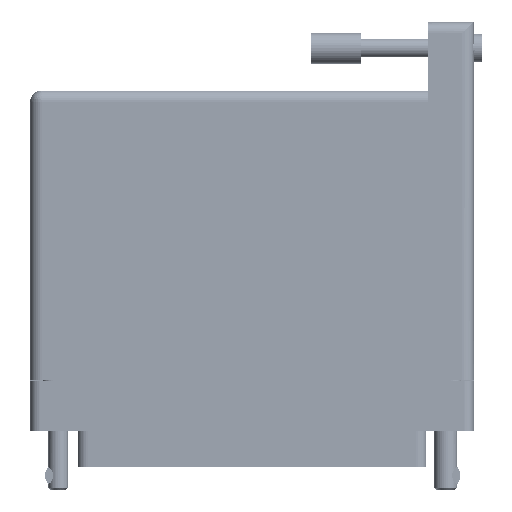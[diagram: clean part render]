
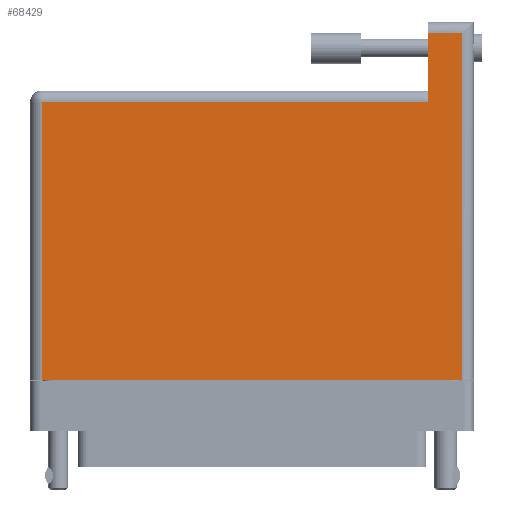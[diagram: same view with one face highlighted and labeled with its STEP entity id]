
A CAD part, front view. The second image highlights one B-rep face of the part: STEP entity #68429.
In plain terms, the highlighted face is planar.
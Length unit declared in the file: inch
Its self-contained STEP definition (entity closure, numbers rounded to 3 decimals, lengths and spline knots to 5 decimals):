
#145 = CARTESIAN_POINT ( 'NONE',  ( -1.359, 1.605, 0.617 ) ) ;
#502 = VERTEX_POINT ( 'NONE', #52005 ) ;
#713 = DIRECTION ( 'NONE',  ( -1., 0., 0. ) ) ;
#2998 = ORIENTED_EDGE ( 'NONE', *, *, #6839, .T. ) ;
#3514 = VECTOR ( 'NONE', #59245, 39.37008 ) ;
#4480 = DIRECTION ( 'NONE',  ( -1., 0., 0. ) ) ;
#5556 = VECTOR ( 'NONE', #54876, 39.37008 ) ;
#6839 = EDGE_CURVE ( 'NONE', #502, #74242, #24138, .T. ) ;
#7007 = CARTESIAN_POINT ( 'NONE',  ( 1.289, 2.095, 0.617 ) ) ;
#7639 = LINE ( 'NONE', #31996, #48152 ) ;
#8585 = LINE ( 'NONE', #68110, #5556 ) ;
#9643 = CARTESIAN_POINT ( 'NONE',  ( 1.289, -0.1, 0.617 ) ) ;
#11271 = DIRECTION ( 'NONE',  ( 0., 0., -1. ) ) ;
#11855 = DIRECTION ( 'NONE',  ( 0., -1., 0. ) ) ;
#16062 = LINE ( 'NONE', #145, #48387 ) ;
#19896 = EDGE_CURVE ( 'NONE', #54878, #42612, #7639, .T. ) ;
#20087 = EDGE_CURVE ( 'NONE', #42612, #45957, #8585, .T. ) ;
#21546 = EDGE_LOOP ( 'NONE', ( #42509, #2998, #46764, #37525, #61223, #74706 ) ) ;
#21786 = EDGE_CURVE ( 'NONE', #60693, #54878, #76334, .T. ) ;
#22994 = CARTESIAN_POINT ( 'NONE',  ( 1.079, 1.605, 0.617 ) ) ;
#24138 = LINE ( 'NONE', #31368, #67548 ) ;
#26674 = EDGE_CURVE ( 'NONE', #45957, #502, #16062, .T. ) ;
#26702 = VECTOR ( 'NONE', #29701, 39.37008 ) ;
#29701 = DIRECTION ( 'NONE',  ( 1., 0., 0. ) ) ;
#29706 = CARTESIAN_POINT ( 'NONE',  ( 1.289, 2.025, 0.617 ) ) ;
#31368 = CARTESIAN_POINT ( 'NONE',  ( -1.289, -0.1, 0.617 ) ) ;
#31996 = CARTESIAN_POINT ( 'NONE',  ( -1.359, 2.025, 0.617 ) ) ;
#37525 = ORIENTED_EDGE ( 'NONE', *, *, #21786, .T. ) ;
#40041 = AXIS2_PLACEMENT_3D ( 'NONE', #62418, #11271, #4480 ) ;
#42080 = CARTESIAN_POINT ( 'NONE',  ( -1.289, -0.1, 0.617 ) ) ;
#42509 = ORIENTED_EDGE ( 'NONE', *, *, #26674, .T. ) ;
#42612 = VERTEX_POINT ( 'NONE', #44245 ) ;
#44245 = CARTESIAN_POINT ( 'NONE',  ( 1.079, 2.025, 0.617 ) ) ;
#45957 = VERTEX_POINT ( 'NONE', #22994 ) ;
#46764 = ORIENTED_EDGE ( 'NONE', *, *, #53523, .T. ) ;
#48152 = VECTOR ( 'NONE', #83414, 39.37008 ) ;
#48387 = VECTOR ( 'NONE', #713, 39.37008 ) ;
#52005 = CARTESIAN_POINT ( 'NONE',  ( -1.289, 1.605, 0.617 ) ) ;
#53523 = EDGE_CURVE ( 'NONE', #74242, #60693, #71150, .T. ) ;
#54876 = DIRECTION ( 'NONE',  ( 0., -1., 0. ) ) ;
#54878 = VERTEX_POINT ( 'NONE', #29706 ) ;
#55146 = CARTESIAN_POINT ( 'NONE',  ( -1.359, -0.1, 0.617 ) ) ;
#59245 = DIRECTION ( 'NONE',  ( 0., 1., 0. ) ) ;
#60693 = VERTEX_POINT ( 'NONE', #9643 ) ;
#61223 = ORIENTED_EDGE ( 'NONE', *, *, #19896, .T. ) ;
#62418 = CARTESIAN_POINT ( 'NONE',  ( -1.359, 1.675, 0.617 ) ) ;
#67548 = VECTOR ( 'NONE', #11855, 39.37008 ) ;
#68110 = CARTESIAN_POINT ( 'NONE',  ( 1.079, 2.095, 0.617 ) ) ;
#68429 = ADVANCED_FACE ( 'NONE', ( #70540 ), #74872, .F. ) ;
#70540 = FACE_OUTER_BOUND ( 'NONE', #21546, .T. ) ;
#71150 = LINE ( 'NONE', #55146, #26702 ) ;
#74242 = VERTEX_POINT ( 'NONE', #42080 ) ;
#74706 = ORIENTED_EDGE ( 'NONE', *, *, #20087, .T. ) ;
#74872 = PLANE ( 'NONE',  #40041 ) ;
#76334 = LINE ( 'NONE', #7007, #3514 ) ;
#83414 = DIRECTION ( 'NONE',  ( -1., 0., 0. ) ) ;
